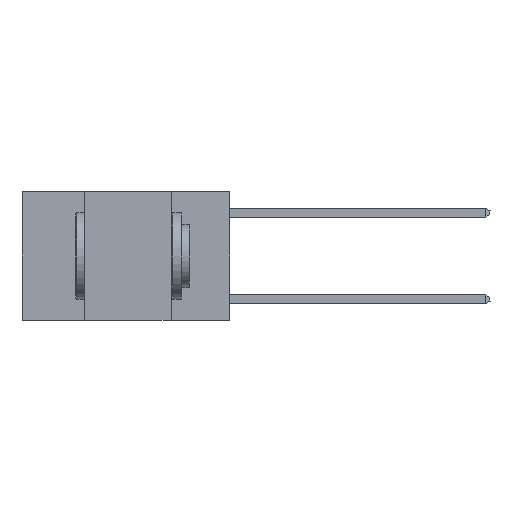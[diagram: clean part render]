
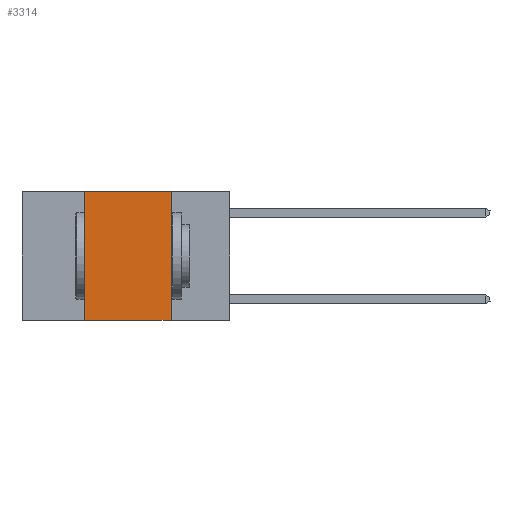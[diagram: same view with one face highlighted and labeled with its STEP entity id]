
A CAD part, left-side view. The second image highlights one B-rep face of the part: STEP entity #3314.
In plain terms, the highlighted planar face has unit normal (-1, 0, 0).
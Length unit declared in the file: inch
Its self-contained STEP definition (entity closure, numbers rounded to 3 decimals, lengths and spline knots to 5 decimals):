
#512 = ORIENTED_EDGE ( 'NONE', *, *, #11667, .F. ) ;
#523 = EDGE_CURVE ( 'NONE', #5055, #7029, #21171, .T. ) ;
#945 = ORIENTED_EDGE ( 'NONE', *, *, #4116, .T. ) ;
#2112 = VECTOR ( 'NONE', #18326, 39.37008 ) ;
#2491 = VECTOR ( 'NONE', #16075, 39.37008 ) ;
#2527 = DIRECTION ( 'NONE',  ( 1., 0., 0. ) ) ;
#3314 = ADVANCED_FACE ( 'NONE', ( #13006 ), #17729, .F. ) ;
#3528 = CARTESIAN_POINT ( 'NONE',  ( 0., 0.6, 0. ) ) ;
#3563 = VERTEX_POINT ( 'NONE', #13974 ) ;
#3680 = AXIS2_PLACEMENT_3D ( 'NONE', #6001, #2527, #9339 ) ;
#4116 = EDGE_CURVE ( 'NONE', #3563, #7029, #12020, .T. ) ;
#4618 = CARTESIAN_POINT ( 'NONE',  ( 0., 0.17, 0. ) ) ;
#5055 = VERTEX_POINT ( 'NONE', #11861 ) ;
#6001 = CARTESIAN_POINT ( 'NONE',  ( 0., 0.6, 0. ) ) ;
#6156 = CARTESIAN_POINT ( 'NONE',  ( 0., 0.42, 0. ) ) ;
#6164 = DIRECTION ( 'NONE',  ( 0., -1., 0. ) ) ;
#7029 = VERTEX_POINT ( 'NONE', #8143 ) ;
#7068 = VERTEX_POINT ( 'NONE', #6156 ) ;
#8143 = CARTESIAN_POINT ( 'NONE',  ( 0., 0.17, -0.37 ) ) ;
#8151 = CARTESIAN_POINT ( 'NONE',  ( 0., 0.6, -0.37 ) ) ;
#9339 = DIRECTION ( 'NONE',  ( 0., 0., -1. ) ) ;
#10225 = LINE ( 'NONE', #3528, #2112 ) ;
#10800 = EDGE_LOOP ( 'NONE', ( #19920, #21568, #512, #945 ) ) ;
#10824 = CARTESIAN_POINT ( 'NONE',  ( 0., 0.42, 0. ) ) ;
#11044 = DIRECTION ( 'NONE',  ( 0., 0., 1. ) ) ;
#11667 = EDGE_CURVE ( 'NONE', #3563, #7068, #12287, .T. ) ;
#11861 = CARTESIAN_POINT ( 'NONE',  ( 0., 0.17, 0. ) ) ;
#12020 = LINE ( 'NONE', #8151, #20050 ) ;
#12287 = LINE ( 'NONE', #10824, #12765 ) ;
#12435 = EDGE_CURVE ( 'NONE', #7068, #5055, #10225, .T. ) ;
#12765 = VECTOR ( 'NONE', #11044, 39.37008 ) ;
#13006 = FACE_OUTER_BOUND ( 'NONE', #10800, .T. ) ;
#13974 = CARTESIAN_POINT ( 'NONE',  ( 0., 0.42, -0.37 ) ) ;
#16075 = DIRECTION ( 'NONE',  ( 0., 0., -1. ) ) ;
#17729 = PLANE ( 'NONE',  #3680 ) ;
#18326 = DIRECTION ( 'NONE',  ( 0., -1., 0. ) ) ;
#19920 = ORIENTED_EDGE ( 'NONE', *, *, #523, .F. ) ;
#20050 = VECTOR ( 'NONE', #6164, 39.37008 ) ;
#21171 = LINE ( 'NONE', #4618, #2491 ) ;
#21568 = ORIENTED_EDGE ( 'NONE', *, *, #12435, .F. ) ;
